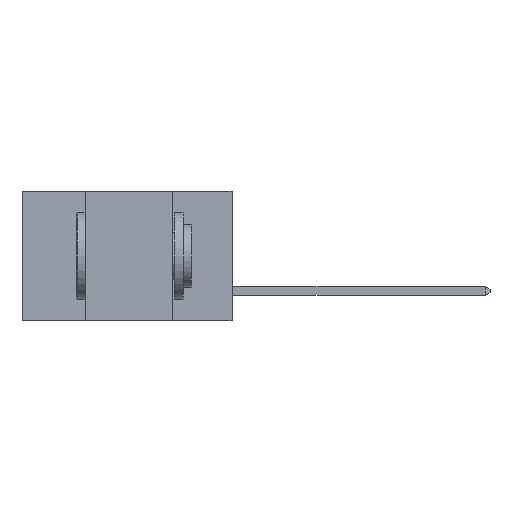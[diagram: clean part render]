
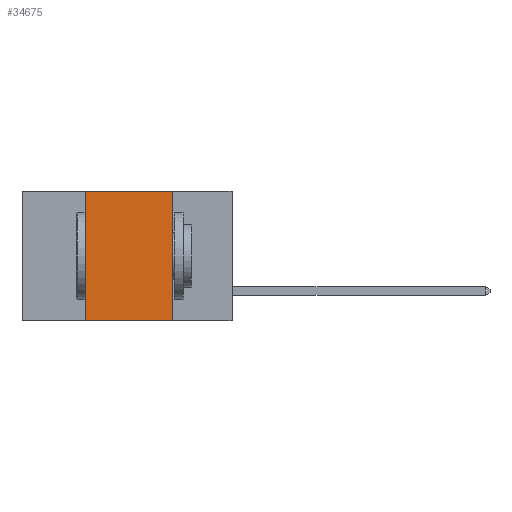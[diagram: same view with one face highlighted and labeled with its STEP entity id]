
A CAD part, left-side view. The second image highlights one B-rep face of the part: STEP entity #34675.
In plain terms, the highlighted planar face has unit normal (-1, 0, 0).
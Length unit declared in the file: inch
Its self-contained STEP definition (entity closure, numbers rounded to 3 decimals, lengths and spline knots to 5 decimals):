
#48 = DIRECTION ( 'NONE',  ( 0., 0., -1. ) ) ;
#261 = AXIS2_PLACEMENT_3D ( 'NONE', #24930, #25069, #22013 ) ;
#1281 = CARTESIAN_POINT ( 'NONE',  ( 0., 0.17, -0.37 ) ) ;
#2125 = CARTESIAN_POINT ( 'NONE',  ( 0., 0.17, 0. ) ) ;
#2324 = CARTESIAN_POINT ( 'NONE',  ( 0., 0.6, 0. ) ) ;
#3683 = LINE ( 'NONE', #8704, #18102 ) ;
#7259 = ORIENTED_EDGE ( 'NONE', *, *, #24992, .F. ) ;
#8704 = CARTESIAN_POINT ( 'NONE',  ( 0., 0.42, 0. ) ) ;
#11206 = ORIENTED_EDGE ( 'NONE', *, *, #23982, .T. ) ;
#12501 = CARTESIAN_POINT ( 'NONE',  ( 0., 0.6, -0.37 ) ) ;
#12528 = CARTESIAN_POINT ( 'NONE',  ( 0., 0.17, 0. ) ) ;
#13408 = VECTOR ( 'NONE', #31049, 39.37008 ) ;
#14788 = EDGE_LOOP ( 'NONE', ( #19478, #26599, #7259, #11206 ) ) ;
#17653 = CARTESIAN_POINT ( 'NONE',  ( 0., 0.42, 0. ) ) ;
#18102 = VECTOR ( 'NONE', #21576, 39.37008 ) ;
#18563 = VERTEX_POINT ( 'NONE', #1281 ) ;
#19266 = CARTESIAN_POINT ( 'NONE',  ( 0., 0.42, -0.37 ) ) ;
#19478 = ORIENTED_EDGE ( 'NONE', *, *, #31098, .F. ) ;
#19558 = VERTEX_POINT ( 'NONE', #19266 ) ;
#21576 = DIRECTION ( 'NONE',  ( 0., 0., 1. ) ) ;
#22013 = DIRECTION ( 'NONE',  ( 0., 0., -1. ) ) ;
#22083 = DIRECTION ( 'NONE',  ( 0., -1., 0. ) ) ;
#23598 = FACE_OUTER_BOUND ( 'NONE', #14788, .T. ) ;
#23982 = EDGE_CURVE ( 'NONE', #19558, #18563, #31627, .T. ) ;
#24337 = VECTOR ( 'NONE', #48, 39.37008 ) ;
#24930 = CARTESIAN_POINT ( 'NONE',  ( 0., 0.6, 0. ) ) ;
#24992 = EDGE_CURVE ( 'NONE', #19558, #27258, #3683, .T. ) ;
#25069 = DIRECTION ( 'NONE',  ( 1., 0., 0. ) ) ;
#26599 = ORIENTED_EDGE ( 'NONE', *, *, #37140, .F. ) ;
#27258 = VERTEX_POINT ( 'NONE', #17653 ) ;
#31049 = DIRECTION ( 'NONE',  ( 0., -1., 0. ) ) ;
#31098 = EDGE_CURVE ( 'NONE', #32064, #18563, #33239, .T. ) ;
#31627 = LINE ( 'NONE', #12501, #39043 ) ;
#32064 = VERTEX_POINT ( 'NONE', #2125 ) ;
#33239 = LINE ( 'NONE', #12528, #24337 ) ;
#34675 = ADVANCED_FACE ( 'NONE', ( #23598 ), #40831, .F. ) ;
#35248 = LINE ( 'NONE', #2324, #13408 ) ;
#37140 = EDGE_CURVE ( 'NONE', #27258, #32064, #35248, .T. ) ;
#39043 = VECTOR ( 'NONE', #22083, 39.37008 ) ;
#40831 = PLANE ( 'NONE',  #261 ) ;
